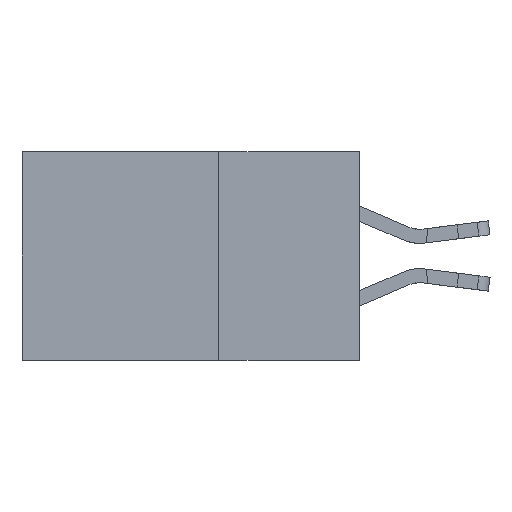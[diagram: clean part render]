
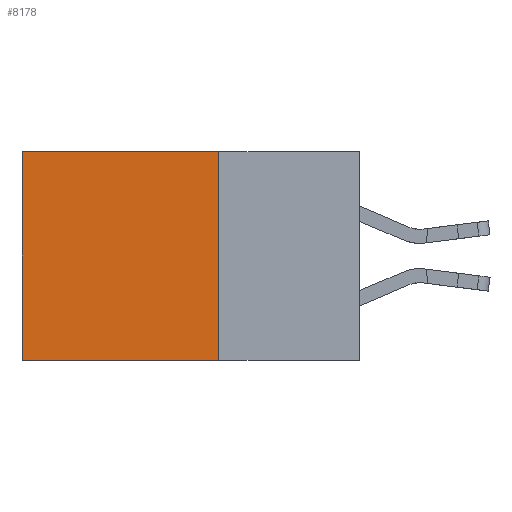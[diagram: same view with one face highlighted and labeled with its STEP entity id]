
A CAD part, left-side view. The second image highlights one B-rep face of the part: STEP entity #8178.
In plain terms, the highlighted planar face has unit normal (-1, 0, 0).
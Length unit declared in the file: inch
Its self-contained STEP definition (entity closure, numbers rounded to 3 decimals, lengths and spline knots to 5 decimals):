
#63 = CARTESIAN_POINT ( 'NONE',  ( 0.2875, 0.25, 0. ) ) ;
#1321 = ORIENTED_EDGE ( 'NONE', *, *, #17931, .F. ) ;
#1368 = CARTESIAN_POINT ( 'NONE',  ( 0.2875, 0.6, 0. ) ) ;
#1696 = LINE ( 'NONE', #11663, #25625 ) ;
#6473 = CARTESIAN_POINT ( 'NONE',  ( 0.2875, 0.25, 0. ) ) ;
#6972 = ORIENTED_EDGE ( 'NONE', *, *, #26149, .F. ) ;
#7532 = EDGE_CURVE ( 'NONE', #19583, #22432, #23821, .T. ) ;
#7649 = PLANE ( 'NONE',  #14220 ) ;
#8178 = ADVANCED_FACE ( 'NONE', ( #17005 ), #7649, .F. ) ;
#9371 = DIRECTION ( 'NONE',  ( 0., 0., -1. ) ) ;
#10033 = CARTESIAN_POINT ( 'NONE',  ( 0.2875, 0.6, 0. ) ) ;
#11192 = VERTEX_POINT ( 'NONE', #6473 ) ;
#11663 = CARTESIAN_POINT ( 'NONE',  ( 0.2875, 0.25, 0. ) ) ;
#13344 = CARTESIAN_POINT ( 'NONE',  ( 0.2875, 0.6, -0.37 ) ) ;
#13763 = ORIENTED_EDGE ( 'NONE', *, *, #7532, .T. ) ;
#14072 = VECTOR ( 'NONE', #21373, 39.37008 ) ;
#14152 = DIRECTION ( 'NONE',  ( 0., 0., -1. ) ) ;
#14220 = AXIS2_PLACEMENT_3D ( 'NONE', #63, #14695, #9371 ) ;
#14695 = DIRECTION ( 'NONE',  ( 1., 0., 0. ) ) ;
#14909 = LINE ( 'NONE', #25741, #19961 ) ;
#17005 = FACE_OUTER_BOUND ( 'NONE', #17963, .T. ) ;
#17538 = VERTEX_POINT ( 'NONE', #21202 ) ;
#17931 = EDGE_CURVE ( 'NONE', #17538, #22432, #19589, .T. ) ;
#17963 = EDGE_LOOP ( 'NONE', ( #13763, #1321, #6972, #29086 ) ) ;
#19583 = VERTEX_POINT ( 'NONE', #1368 ) ;
#19589 = LINE ( 'NONE', #27328, #23506 ) ;
#19961 = VECTOR ( 'NONE', #14152, 39.37008 ) ;
#21202 = CARTESIAN_POINT ( 'NONE',  ( 0.2875, 0.25, -0.37 ) ) ;
#21373 = DIRECTION ( 'NONE',  ( 0., 0., -1. ) ) ;
#22432 = VERTEX_POINT ( 'NONE', #13344 ) ;
#23506 = VECTOR ( 'NONE', #25386, 39.37008 ) ;
#23821 = LINE ( 'NONE', #10033, #14072 ) ;
#25386 = DIRECTION ( 'NONE',  ( 0., 1., 0. ) ) ;
#25625 = VECTOR ( 'NONE', #29743, 39.37008 ) ;
#25741 = CARTESIAN_POINT ( 'NONE',  ( 0.2875, 0.25, 0. ) ) ;
#26149 = EDGE_CURVE ( 'NONE', #11192, #17538, #14909, .T. ) ;
#27328 = CARTESIAN_POINT ( 'NONE',  ( 0.2875, 0.25, -0.37 ) ) ;
#29080 = EDGE_CURVE ( 'NONE', #11192, #19583, #1696, .T. ) ;
#29086 = ORIENTED_EDGE ( 'NONE', *, *, #29080, .T. ) ;
#29743 = DIRECTION ( 'NONE',  ( 0., 1., 0. ) ) ;
